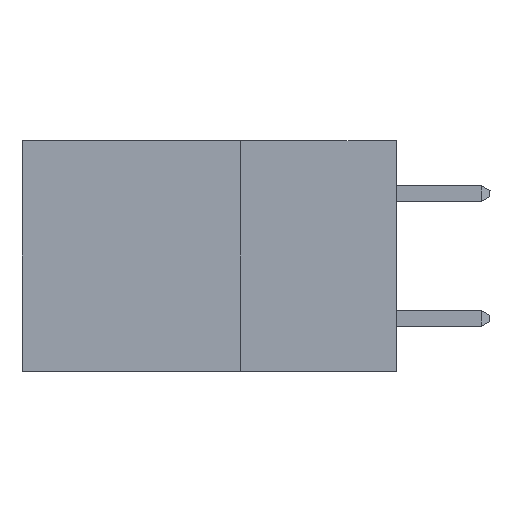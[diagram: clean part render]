
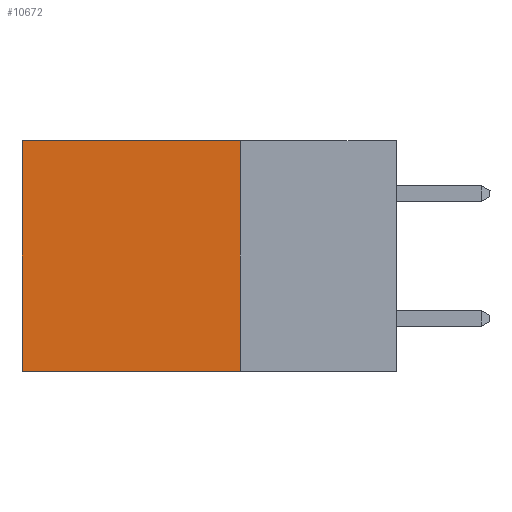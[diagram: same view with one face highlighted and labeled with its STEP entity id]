
A CAD part, left-side view. The second image highlights one B-rep face of the part: STEP entity #10672.
In plain terms, the highlighted planar face has unit normal (-1, 0, 0).
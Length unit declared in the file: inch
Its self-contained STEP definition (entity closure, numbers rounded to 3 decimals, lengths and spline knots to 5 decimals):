
#359 = VECTOR ( 'NONE', #10110, 39.37008 ) ;
#736 = PLANE ( 'NONE',  #1422 ) ;
#1422 = AXIS2_PLACEMENT_3D ( 'NONE', #11844, #9579, #2031 ) ;
#1751 = VECTOR ( 'NONE', #7662, 39.37008 ) ;
#1873 = VERTEX_POINT ( 'NONE', #5487 ) ;
#2031 = DIRECTION ( 'NONE',  ( 0., 0., -1. ) ) ;
#2114 = CARTESIAN_POINT ( 'NONE',  ( 0.298, 0.6, 0. ) ) ;
#3068 = LINE ( 'NONE', #2114, #7269 ) ;
#3384 = EDGE_CURVE ( 'NONE', #1873, #7437, #10006, .T. ) ;
#3499 = EDGE_CURVE ( 'NONE', #7437, #7762, #8497, .T. ) ;
#4001 = ORIENTED_EDGE ( 'NONE', *, *, #3384, .F. ) ;
#4712 = ORIENTED_EDGE ( 'NONE', *, *, #10053, .T. ) ;
#5487 = CARTESIAN_POINT ( 'NONE',  ( 0.298, 0.25, 0. ) ) ;
#7211 = DIRECTION ( 'NONE',  ( 0., 0., -1. ) ) ;
#7269 = VECTOR ( 'NONE', #7211, 39.37008 ) ;
#7437 = VERTEX_POINT ( 'NONE', #10759 ) ;
#7641 = CARTESIAN_POINT ( 'NONE',  ( 0.298, 0.25, 0. ) ) ;
#7662 = DIRECTION ( 'NONE',  ( 0., 1., 0. ) ) ;
#7722 = CARTESIAN_POINT ( 'NONE',  ( 0.298, 0.25, 0. ) ) ;
#7762 = VERTEX_POINT ( 'NONE', #8435 ) ;
#8435 = CARTESIAN_POINT ( 'NONE',  ( 0.298, 0.6, -0.37 ) ) ;
#8497 = LINE ( 'NONE', #13696, #1751 ) ;
#8817 = VECTOR ( 'NONE', #14679, 39.37008 ) ;
#9083 = EDGE_CURVE ( 'NONE', #1873, #14063, #14236, .T. ) ;
#9530 = FACE_OUTER_BOUND ( 'NONE', #10298, .T. ) ;
#9579 = DIRECTION ( 'NONE',  ( 1., 0., 0. ) ) ;
#10006 = LINE ( 'NONE', #7641, #359 ) ;
#10053 = EDGE_CURVE ( 'NONE', #14063, #7762, #3068, .T. ) ;
#10110 = DIRECTION ( 'NONE',  ( 0., 0., -1. ) ) ;
#10298 = EDGE_LOOP ( 'NONE', ( #4712, #10912, #4001, #13540 ) ) ;
#10672 = ADVANCED_FACE ( 'NONE', ( #9530 ), #736, .F. ) ;
#10759 = CARTESIAN_POINT ( 'NONE',  ( 0.298, 0.25, -0.37 ) ) ;
#10912 = ORIENTED_EDGE ( 'NONE', *, *, #3499, .F. ) ;
#11844 = CARTESIAN_POINT ( 'NONE',  ( 0.298, 0.25, 0. ) ) ;
#13540 = ORIENTED_EDGE ( 'NONE', *, *, #9083, .T. ) ;
#13696 = CARTESIAN_POINT ( 'NONE',  ( 0.298, 0.25, -0.37 ) ) ;
#14063 = VERTEX_POINT ( 'NONE', #14504 ) ;
#14236 = LINE ( 'NONE', #7722, #8817 ) ;
#14504 = CARTESIAN_POINT ( 'NONE',  ( 0.298, 0.6, 0. ) ) ;
#14679 = DIRECTION ( 'NONE',  ( 0., 1., 0. ) ) ;
